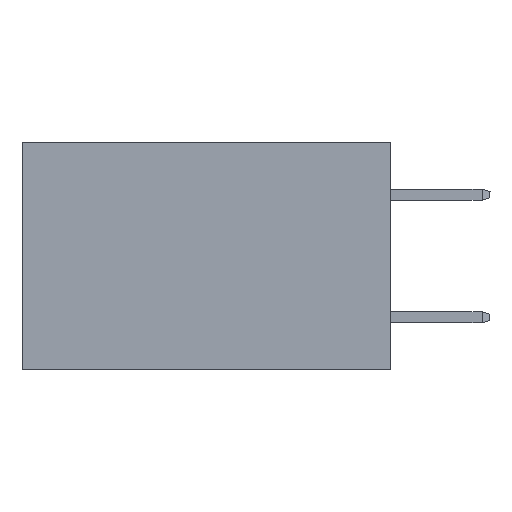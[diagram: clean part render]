
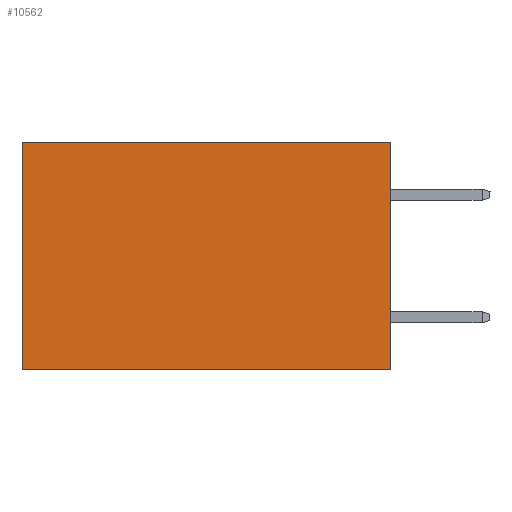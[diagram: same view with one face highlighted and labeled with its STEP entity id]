
A CAD part, left-side view. The second image highlights one B-rep face of the part: STEP entity #10562.
In plain terms, the highlighted planar face has unit normal (-1, 0, 0).
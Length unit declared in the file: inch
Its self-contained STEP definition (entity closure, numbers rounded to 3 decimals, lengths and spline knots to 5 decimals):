
#812 = PLANE ( 'NONE',  #3860 ) ;
#1428 = CARTESIAN_POINT ( 'NONE',  ( 0.2875, 0.6, 0. ) ) ;
#1827 = DIRECTION ( 'NONE',  ( 0., 0., -1. ) ) ;
#1884 = CARTESIAN_POINT ( 'NONE',  ( 0.2875, 0., 0. ) ) ;
#2112 = CARTESIAN_POINT ( 'NONE',  ( 0.2875, 0., -0.37 ) ) ;
#2346 = EDGE_CURVE ( 'NONE', #5661, #2869, #13118, .T. ) ;
#2731 = VECTOR ( 'NONE', #5931, 39.37008 ) ;
#2869 = VERTEX_POINT ( 'NONE', #3670 ) ;
#3670 = CARTESIAN_POINT ( 'NONE',  ( 0.2875, 0.6, -0.37 ) ) ;
#3860 = AXIS2_PLACEMENT_3D ( 'NONE', #1884, #14262, #1827 ) ;
#4050 = VERTEX_POINT ( 'NONE', #7470 ) ;
#4067 = VECTOR ( 'NONE', #10438, 39.37008 ) ;
#4458 = ORIENTED_EDGE ( 'NONE', *, *, #2346, .T. ) ;
#4903 = EDGE_LOOP ( 'NONE', ( #4458, #13659, #7990, #8187 ) ) ;
#5293 = LINE ( 'NONE', #2112, #14459 ) ;
#5661 = VERTEX_POINT ( 'NONE', #1428 ) ;
#5727 = EDGE_CURVE ( 'NONE', #4050, #2869, #5293, .T. ) ;
#5931 = DIRECTION ( 'NONE',  ( 0., 0., -1. ) ) ;
#5951 = EDGE_CURVE ( 'NONE', #10627, #5661, #11590, .T. ) ;
#6789 = DIRECTION ( 'NONE',  ( 0., 0., -1. ) ) ;
#7470 = CARTESIAN_POINT ( 'NONE',  ( 0.2875, 0., -0.37 ) ) ;
#7990 = ORIENTED_EDGE ( 'NONE', *, *, #14295, .F. ) ;
#8187 = ORIENTED_EDGE ( 'NONE', *, *, #5951, .T. ) ;
#9924 = DIRECTION ( 'NONE',  ( 0., 1., 0. ) ) ;
#10017 = LINE ( 'NONE', #13610, #11784 ) ;
#10438 = DIRECTION ( 'NONE',  ( 0., 1., 0. ) ) ;
#10562 = ADVANCED_FACE ( 'NONE', ( #14231 ), #812, .F. ) ;
#10627 = VERTEX_POINT ( 'NONE', #10825 ) ;
#10825 = CARTESIAN_POINT ( 'NONE',  ( 0.2875, 0., 0. ) ) ;
#11590 = LINE ( 'NONE', #13942, #4067 ) ;
#11784 = VECTOR ( 'NONE', #6789, 39.37008 ) ;
#13118 = LINE ( 'NONE', #13904, #2731 ) ;
#13610 = CARTESIAN_POINT ( 'NONE',  ( 0.2875, 0., 0. ) ) ;
#13659 = ORIENTED_EDGE ( 'NONE', *, *, #5727, .F. ) ;
#13904 = CARTESIAN_POINT ( 'NONE',  ( 0.2875, 0.6, 0. ) ) ;
#13942 = CARTESIAN_POINT ( 'NONE',  ( 0.2875, 0., 0. ) ) ;
#14231 = FACE_OUTER_BOUND ( 'NONE', #4903, .T. ) ;
#14262 = DIRECTION ( 'NONE',  ( 1., 0., 0. ) ) ;
#14295 = EDGE_CURVE ( 'NONE', #10627, #4050, #10017, .T. ) ;
#14459 = VECTOR ( 'NONE', #9924, 39.37008 ) ;
